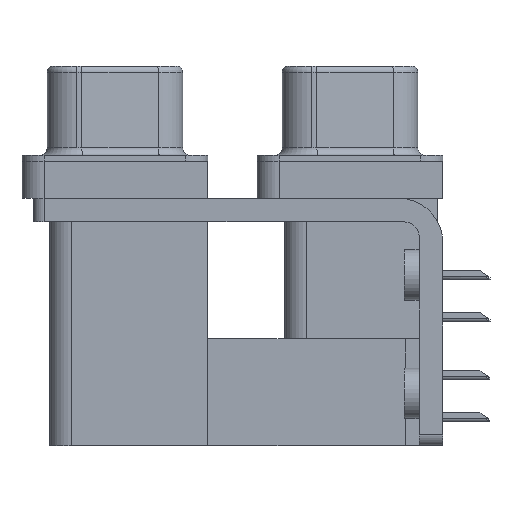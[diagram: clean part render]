
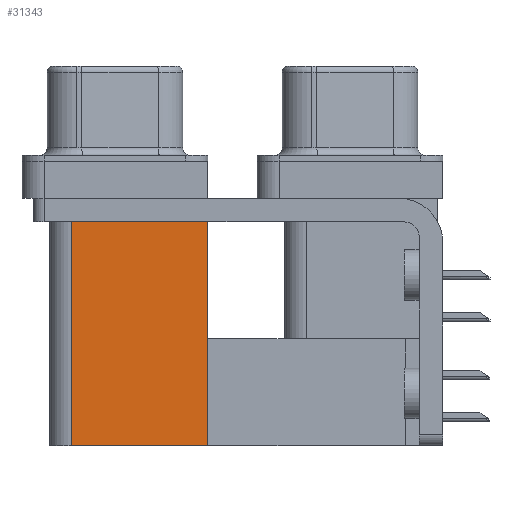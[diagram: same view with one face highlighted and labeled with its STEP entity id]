
A CAD part, left-side view. The second image highlights one B-rep face of the part: STEP entity #31343.
In plain terms, the highlighted planar face has unit normal (-1, 0, 0).
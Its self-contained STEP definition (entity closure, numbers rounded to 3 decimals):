
#7 = PLANE ( 'NONE',  #2660 ) ;
#223 = VECTOR ( 'NONE', #33607, 1000. ) ;
#969 = EDGE_CURVE ( 'NONE', #28847, #1062, #31070, .T. ) ;
#1062 = VERTEX_POINT ( 'NONE', #2780 ) ;
#1733 = CARTESIAN_POINT ( 'NONE',  ( 3.765, 9.6, -2.5 ) ) ;
#2660 = AXIS2_PLACEMENT_3D ( 'NONE', #10492, #7925, #18028 ) ;
#2780 = CARTESIAN_POINT ( 'NONE',  ( 3.765, 18.8, -2.5 ) ) ;
#3060 = ORIENTED_EDGE ( 'NONE', *, *, #25113, .F. ) ;
#3737 = VECTOR ( 'NONE', #4830, 1000. ) ;
#4830 = DIRECTION ( 'NONE',  ( 0., 0., 1. ) ) ;
#6976 = LINE ( 'NONE', #14341, #24310 ) ;
#7925 = DIRECTION ( 'NONE',  ( 1., 0., 0. ) ) ;
#8098 = CARTESIAN_POINT ( 'NONE',  ( 3.765, 9.6, -19.2 ) ) ;
#8585 = EDGE_LOOP ( 'NONE', ( #32980, #3060, #9028, #31043 ) ) ;
#9028 = ORIENTED_EDGE ( 'NONE', *, *, #10278, .F. ) ;
#10278 = EDGE_CURVE ( 'NONE', #21394, #27890, #20613, .T. ) ;
#10492 = CARTESIAN_POINT ( 'NONE',  ( 3.765, 9.6, -19.2 ) ) ;
#10692 = DIRECTION ( 'NONE',  ( 0., 1., 0. ) ) ;
#11613 = DIRECTION ( 'NONE',  ( 0., 0., 1. ) ) ;
#11929 = CARTESIAN_POINT ( 'NONE',  ( 3.765, 9.6, -19.2 ) ) ;
#12723 = CARTESIAN_POINT ( 'NONE',  ( 3.765, 9.6, -19.2 ) ) ;
#14341 = CARTESIAN_POINT ( 'NONE',  ( 3.765, 18.8, -19.2 ) ) ;
#17803 = VECTOR ( 'NONE', #10692, 1000. ) ;
#18028 = DIRECTION ( 'NONE',  ( 0., 0., -1. ) ) ;
#20613 = LINE ( 'NONE', #8098, #223 ) ;
#20934 = FACE_OUTER_BOUND ( 'NONE', #8585, .T. ) ;
#21394 = VERTEX_POINT ( 'NONE', #11929 ) ;
#24310 = VECTOR ( 'NONE', #11613, 1000. ) ;
#25113 = EDGE_CURVE ( 'NONE', #27890, #1062, #6976, .T. ) ;
#26093 = CARTESIAN_POINT ( 'NONE',  ( 3.765, 9.6, -2.5 ) ) ;
#27890 = VERTEX_POINT ( 'NONE', #29982 ) ;
#28847 = VERTEX_POINT ( 'NONE', #1733 ) ;
#29982 = CARTESIAN_POINT ( 'NONE',  ( 3.765, 18.8, -19.2 ) ) ;
#31043 = ORIENTED_EDGE ( 'NONE', *, *, #31255, .T. ) ;
#31070 = LINE ( 'NONE', #26093, #17803 ) ;
#31203 = LINE ( 'NONE', #12723, #3737 ) ;
#31255 = EDGE_CURVE ( 'NONE', #21394, #28847, #31203, .T. ) ;
#31343 = ADVANCED_FACE ( 'NONE', ( #20934 ), #7, .F. ) ;
#32980 = ORIENTED_EDGE ( 'NONE', *, *, #969, .T. ) ;
#33607 = DIRECTION ( 'NONE',  ( 0., 1., 0. ) ) ;
